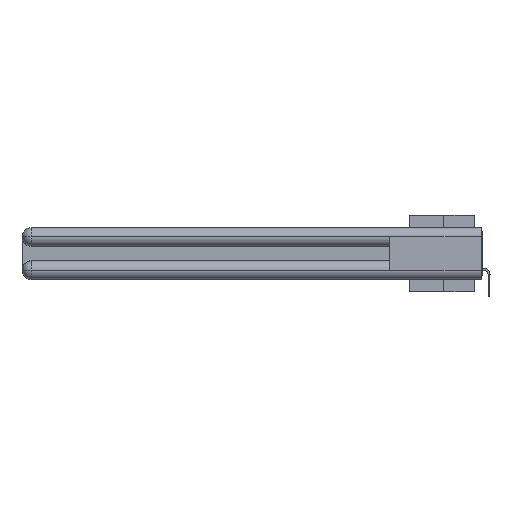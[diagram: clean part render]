
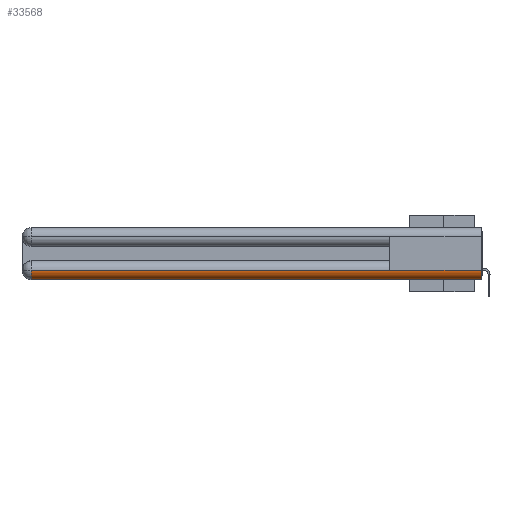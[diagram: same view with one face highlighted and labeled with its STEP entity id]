
A CAD part, left-side view. The second image highlights one B-rep face of the part: STEP entity #33568.
In plain terms, the highlighted cylindrical face has radius 1.562 mm (diameter 3.124 mm), a partial arc.
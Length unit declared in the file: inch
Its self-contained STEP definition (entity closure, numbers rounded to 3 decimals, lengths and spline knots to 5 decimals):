
#369 = EDGE_CURVE ( 'NONE', #17929, #10675, #37363, .T. ) ;
#1857 = ORIENTED_EDGE ( 'NONE', *, *, #369, .T. ) ;
#2829 = CARTESIAN_POINT ( 'NONE',  ( 0., 0., -0.2785 ) ) ;
#3504 = ORIENTED_EDGE ( 'NONE', *, *, #6197, .F. ) ;
#4946 = EDGE_LOOP ( 'NONE', ( #1857, #17311, #3504, #36105, #5733 ) ) ;
#5733 = ORIENTED_EDGE ( 'NONE', *, *, #10251, .F. ) ;
#6197 = EDGE_CURVE ( 'NONE', #27539, #15867, #20677, .T. ) ;
#7926 = CARTESIAN_POINT ( 'NONE',  ( 0.0615, 0., -0.34 ) ) ;
#9264 = CIRCLE ( 'NONE', #29685, 0.0615 ) ;
#10217 = CARTESIAN_POINT ( 'NONE',  ( 0.0615, 2.94, -0.2785 ) ) ;
#10251 = EDGE_CURVE ( 'NONE', #17929, #33219, #17437, .T. ) ;
#10670 = CARTESIAN_POINT ( 'NONE',  ( 0., 0., -0.2785 ) ) ;
#10675 = VERTEX_POINT ( 'NONE', #31988 ) ;
#11193 = EDGE_CURVE ( 'NONE', #33219, #27539, #9264, .T. ) ;
#12804 = CARTESIAN_POINT ( 'NONE',  ( 0.0615, 0., -0.34 ) ) ;
#14167 = CIRCLE ( 'NONE', #18044, 0.0615 ) ;
#14256 = DIRECTION ( 'NONE',  ( 0., -1., 0. ) ) ;
#15867 = VERTEX_POINT ( 'NONE', #23201 ) ;
#17311 = ORIENTED_EDGE ( 'NONE', *, *, #26241, .T. ) ;
#17437 = LINE ( 'NONE', #10670, #29626 ) ;
#17929 = VERTEX_POINT ( 'NONE', #22922 ) ;
#18044 = AXIS2_PLACEMENT_3D ( 'NONE', #10217, #22395, #36967 ) ;
#19815 = FACE_OUTER_BOUND ( 'NONE', #4946, .T. ) ;
#19991 = AXIS2_PLACEMENT_3D ( 'NONE', #38578, #34986, #20208 ) ;
#20208 = DIRECTION ( 'NONE',  ( 0., 0., -1. ) ) ;
#20677 = LINE ( 'NONE', #7926, #29458 ) ;
#21584 = DIRECTION ( 'NONE',  ( 0., 1., 0. ) ) ;
#22395 = DIRECTION ( 'NONE',  ( 0., -1., 0. ) ) ;
#22922 = CARTESIAN_POINT ( 'NONE',  ( 0., 0.6, -0.2785 ) ) ;
#23201 = CARTESIAN_POINT ( 'NONE',  ( 0.0615, 2.94, -0.34 ) ) ;
#23930 = CARTESIAN_POINT ( 'NONE',  ( 0.0615, 0., -0.2785 ) ) ;
#24990 = CARTESIAN_POINT ( 'NONE',  ( 0., 0., -0.2785 ) ) ;
#25628 = CYLINDRICAL_SURFACE ( 'NONE', #19991, 0.0615 ) ;
#26241 = EDGE_CURVE ( 'NONE', #10675, #15867, #14167, .T. ) ;
#27120 = DIRECTION ( 'NONE',  ( 0., -1., 0. ) ) ;
#27539 = VERTEX_POINT ( 'NONE', #12804 ) ;
#27738 = VECTOR ( 'NONE', #21584, 39.37008 ) ;
#29458 = VECTOR ( 'NONE', #35675, 39.37008 ) ;
#29626 = VECTOR ( 'NONE', #14256, 39.37008 ) ;
#29685 = AXIS2_PLACEMENT_3D ( 'NONE', #23930, #27120, #33120 ) ;
#31988 = CARTESIAN_POINT ( 'NONE',  ( 0., 2.94, -0.2785 ) ) ;
#33120 = DIRECTION ( 'NONE',  ( 1., 0., 0. ) ) ;
#33219 = VERTEX_POINT ( 'NONE', #2829 ) ;
#33568 = ADVANCED_FACE ( 'NONE', ( #19815 ), #25628, .T. ) ;
#34986 = DIRECTION ( 'NONE',  ( 0., -1., 0. ) ) ;
#35675 = DIRECTION ( 'NONE',  ( 0., 1., 0. ) ) ;
#36105 = ORIENTED_EDGE ( 'NONE', *, *, #11193, .F. ) ;
#36967 = DIRECTION ( 'NONE',  ( 0., 0., 1. ) ) ;
#37363 = LINE ( 'NONE', #24990, #27738 ) ;
#38578 = CARTESIAN_POINT ( 'NONE',  ( 0.0615, 0., -0.2785 ) ) ;
